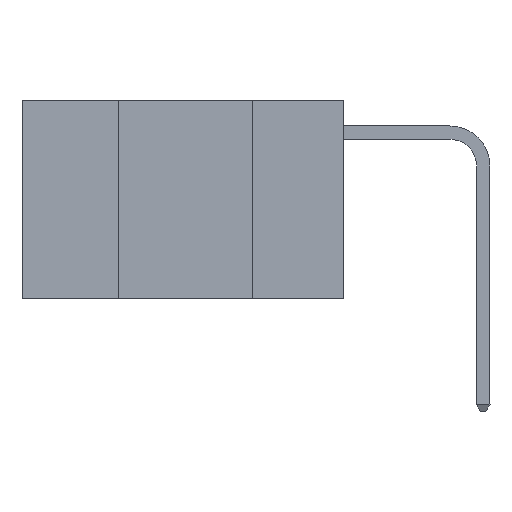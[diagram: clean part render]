
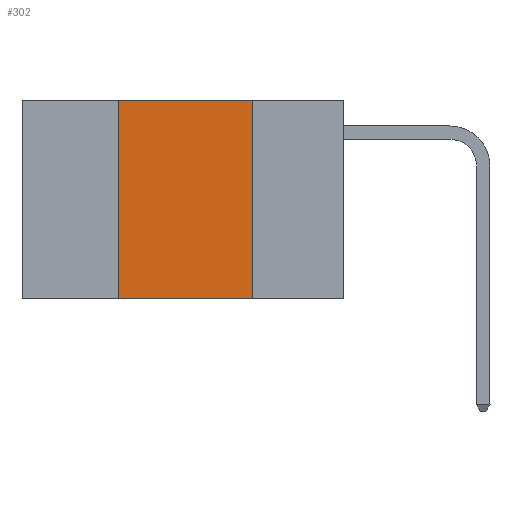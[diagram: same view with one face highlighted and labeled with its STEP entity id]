
A CAD part, left-side view. The second image highlights one B-rep face of the part: STEP entity #302.
In plain terms, the highlighted planar face has unit normal (-1, 0, 0).
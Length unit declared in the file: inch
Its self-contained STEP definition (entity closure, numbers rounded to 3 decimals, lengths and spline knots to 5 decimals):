
#302 = ADVANCED_FACE ( 'NONE', ( #13858 ), #11489, .F. ) ;
#375 = ORIENTED_EDGE ( 'NONE', *, *, #14302, .T. ) ;
#804 = CARTESIAN_POINT ( 'NONE',  ( 0., 0.6, 0. ) ) ;
#1037 = DIRECTION ( 'NONE',  ( 1., 0., 0. ) ) ;
#2623 = CARTESIAN_POINT ( 'NONE',  ( 0., 0.17, -0.37 ) ) ;
#2726 = EDGE_LOOP ( 'NONE', ( #10679, #12377, #10945, #375 ) ) ;
#3476 = VERTEX_POINT ( 'NONE', #8376 ) ;
#4222 = LINE ( 'NONE', #6347, #11593 ) ;
#4355 = CARTESIAN_POINT ( 'NONE',  ( 0., 0.17, 0. ) ) ;
#4442 = VECTOR ( 'NONE', #7886, 39.37008 ) ;
#4743 = LINE ( 'NONE', #9331, #12446 ) ;
#5727 = DIRECTION ( 'NONE',  ( 0., 0., 1. ) ) ;
#5753 = CARTESIAN_POINT ( 'NONE',  ( 0., 0.6, 0. ) ) ;
#6347 = CARTESIAN_POINT ( 'NONE',  ( 0., 0.6, -0.37 ) ) ;
#6503 = DIRECTION ( 'NONE',  ( 0., -1., 0. ) ) ;
#6548 = EDGE_CURVE ( 'NONE', #10309, #10291, #4743, .T. ) ;
#6567 = LINE ( 'NONE', #4355, #10510 ) ;
#7886 = DIRECTION ( 'NONE',  ( 0., -1., 0. ) ) ;
#8376 = CARTESIAN_POINT ( 'NONE',  ( 0., 0.17, 0. ) ) ;
#8822 = LINE ( 'NONE', #804, #4442 ) ;
#8858 = EDGE_CURVE ( 'NONE', #10291, #3476, #8822, .T. ) ;
#9242 = EDGE_CURVE ( 'NONE', #3476, #12927, #6567, .T. ) ;
#9280 = DIRECTION ( 'NONE',  ( 0., 0., -1. ) ) ;
#9331 = CARTESIAN_POINT ( 'NONE',  ( 0., 0.42, 0. ) ) ;
#9335 = CARTESIAN_POINT ( 'NONE',  ( 0., 0.42, 0. ) ) ;
#10104 = AXIS2_PLACEMENT_3D ( 'NONE', #5753, #1037, #9280 ) ;
#10291 = VERTEX_POINT ( 'NONE', #9335 ) ;
#10309 = VERTEX_POINT ( 'NONE', #11703 ) ;
#10510 = VECTOR ( 'NONE', #13466, 39.37008 ) ;
#10679 = ORIENTED_EDGE ( 'NONE', *, *, #9242, .F. ) ;
#10945 = ORIENTED_EDGE ( 'NONE', *, *, #6548, .F. ) ;
#11489 = PLANE ( 'NONE',  #10104 ) ;
#11593 = VECTOR ( 'NONE', #6503, 39.37008 ) ;
#11703 = CARTESIAN_POINT ( 'NONE',  ( 0., 0.42, -0.37 ) ) ;
#12377 = ORIENTED_EDGE ( 'NONE', *, *, #8858, .F. ) ;
#12446 = VECTOR ( 'NONE', #5727, 39.37008 ) ;
#12927 = VERTEX_POINT ( 'NONE', #2623 ) ;
#13466 = DIRECTION ( 'NONE',  ( 0., 0., -1. ) ) ;
#13858 = FACE_OUTER_BOUND ( 'NONE', #2726, .T. ) ;
#14302 = EDGE_CURVE ( 'NONE', #10309, #12927, #4222, .T. ) ;
